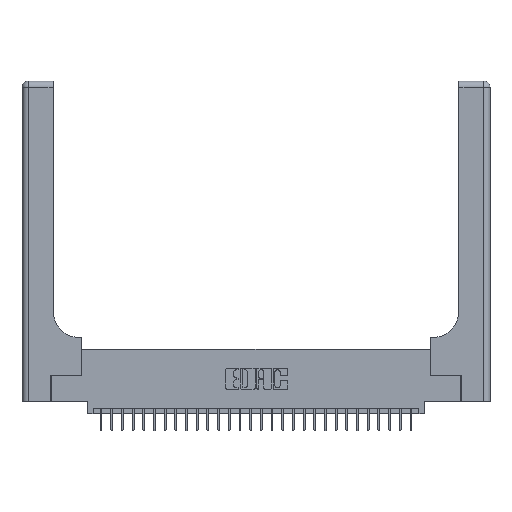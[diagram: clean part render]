
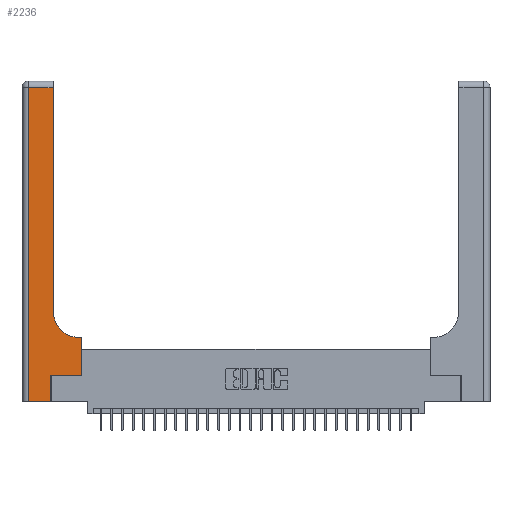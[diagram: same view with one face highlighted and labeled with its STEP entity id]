
A CAD part, top view. The second image highlights one B-rep face of the part: STEP entity #2236.
In plain terms, the highlighted planar face has unit normal (0, 0, 1).
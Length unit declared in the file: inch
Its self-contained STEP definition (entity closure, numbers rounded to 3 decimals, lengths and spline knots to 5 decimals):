
#291 = CARTESIAN_POINT ( 'NONE',  ( 0.06, 2.94, 0.37 ) ) ;
#898 = AXIS2_PLACEMENT_3D ( 'NONE', #12457, #946, #17420 ) ;
#946 = DIRECTION ( 'NONE',  ( 0., 0., -1. ) ) ;
#1152 = CARTESIAN_POINT ( 'NONE',  ( 0.2915, 3., 0.37 ) ) ;
#1405 = CARTESIAN_POINT ( 'NONE',  ( 0.5415, 0.85, 0.37 ) ) ;
#1659 = VECTOR ( 'NONE', #20168, 39.37008 ) ;
#1899 = VERTEX_POINT ( 'NONE', #24719 ) ;
#2165 = LINE ( 'NONE', #14257, #13941 ) ;
#2236 = ADVANCED_FACE ( 'NONE', ( #24741 ), #10393, .F. ) ;
#2517 = LINE ( 'NONE', #11486, #26872 ) ;
#3810 = LINE ( 'NONE', #1152, #28166 ) ;
#3824 = ORIENTED_EDGE ( 'NONE', *, *, #6920, .T. ) ;
#4159 = CARTESIAN_POINT ( 'NONE',  ( 0.269, 0., 0.37 ) ) ;
#4293 = VERTEX_POINT ( 'NONE', #10146 ) ;
#5376 = VERTEX_POINT ( 'NONE', #9492 ) ;
#5674 = EDGE_CURVE ( 'NONE', #18499, #5376, #29000, .T. ) ;
#6738 = EDGE_CURVE ( 'NONE', #12091, #18499, #14197, .T. ) ;
#6920 = EDGE_CURVE ( 'NONE', #1899, #4293, #24886, .T. ) ;
#7078 = DIRECTION ( 'NONE',  ( -1., 0., 0. ) ) ;
#7262 = ORIENTED_EDGE ( 'NONE', *, *, #26365, .T. ) ;
#7520 = EDGE_CURVE ( 'NONE', #28595, #15512, #10056, .T. ) ;
#7571 = CIRCLE ( 'NONE', #26254, 0.25 ) ;
#7953 = CARTESIAN_POINT ( 'NONE',  ( 0.2915, 2.94, 0.37 ) ) ;
#8216 = EDGE_LOOP ( 'NONE', ( #27135, #19461, #10935, #9343, #7262, #21477, #20419, #3824, #23990 ) ) ;
#8591 = DIRECTION ( 'NONE',  ( 1., 0., 0. ) ) ;
#9134 = CARTESIAN_POINT ( 'NONE',  ( 0.269, 0.25, 0.37 ) ) ;
#9343 = ORIENTED_EDGE ( 'NONE', *, *, #10621, .T. ) ;
#9492 = CARTESIAN_POINT ( 'NONE',  ( 0.06, 0., 0.37 ) ) ;
#10056 = LINE ( 'NONE', #9134, #20399 ) ;
#10146 = CARTESIAN_POINT ( 'NONE',  ( 0.5415, 0.6, 0.37 ) ) ;
#10393 = PLANE ( 'NONE',  #898 ) ;
#10621 = EDGE_CURVE ( 'NONE', #5376, #24011, #2165, .T. ) ;
#10935 = ORIENTED_EDGE ( 'NONE', *, *, #5674, .T. ) ;
#11486 = CARTESIAN_POINT ( 'NONE',  ( 0.5585, 0.25, 0.37 ) ) ;
#11944 = DIRECTION ( 'NONE',  ( 1., 0., 0. ) ) ;
#12091 = VERTEX_POINT ( 'NONE', #7953 ) ;
#12300 = VECTOR ( 'NONE', #7078, 39.37008 ) ;
#12457 = CARTESIAN_POINT ( 'NONE',  ( 0., 3., 0.37 ) ) ;
#13941 = VECTOR ( 'NONE', #11944, 39.37008 ) ;
#14134 = EDGE_CURVE ( 'NONE', #15769, #12091, #3810, .T. ) ;
#14197 = LINE ( 'NONE', #17809, #1659 ) ;
#14257 = CARTESIAN_POINT ( 'NONE',  ( 0., 0., 0.37 ) ) ;
#14603 = CARTESIAN_POINT ( 'NONE',  ( 0.06, 3., 0.37 ) ) ;
#15121 = CARTESIAN_POINT ( 'NONE',  ( 0.2915, 0.85, 0.37 ) ) ;
#15512 = VERTEX_POINT ( 'NONE', #30326 ) ;
#15769 = VERTEX_POINT ( 'NONE', #15121 ) ;
#16959 = DIRECTION ( 'NONE',  ( 0., -1., 0. ) ) ;
#17420 = DIRECTION ( 'NONE',  ( -1., 0., 0. ) ) ;
#17809 = CARTESIAN_POINT ( 'NONE',  ( 0., 2.94, 0.37 ) ) ;
#18499 = VERTEX_POINT ( 'NONE', #291 ) ;
#19461 = ORIENTED_EDGE ( 'NONE', *, *, #6738, .T. ) ;
#19994 = DIRECTION ( 'NONE',  ( 0., 1., 0. ) ) ;
#20168 = DIRECTION ( 'NONE',  ( -1., 0., 0. ) ) ;
#20399 = VECTOR ( 'NONE', #26375, 39.37008 ) ;
#20416 = EDGE_CURVE ( 'NONE', #4293, #15769, #7571, .T. ) ;
#20419 = ORIENTED_EDGE ( 'NONE', *, *, #29817, .T. ) ;
#21477 = ORIENTED_EDGE ( 'NONE', *, *, #7520, .T. ) ;
#22551 = CARTESIAN_POINT ( 'NONE',  ( 0.269, 0.25, 0.37 ) ) ;
#23773 = CARTESIAN_POINT ( 'NONE',  ( 0.2915, 0.6, 0.37 ) ) ;
#23813 = VECTOR ( 'NONE', #16959, 39.37008 ) ;
#23990 = ORIENTED_EDGE ( 'NONE', *, *, #20416, .T. ) ;
#24011 = VERTEX_POINT ( 'NONE', #28501 ) ;
#24102 = LINE ( 'NONE', #4159, #30395 ) ;
#24719 = CARTESIAN_POINT ( 'NONE',  ( 0.5585, 0.6, 0.37 ) ) ;
#24741 = FACE_OUTER_BOUND ( 'NONE', #8216, .T. ) ;
#24886 = LINE ( 'NONE', #23773, #12300 ) ;
#26254 = AXIS2_PLACEMENT_3D ( 'NONE', #1405, #29949, #8591 ) ;
#26365 = EDGE_CURVE ( 'NONE', #24011, #28595, #24102, .T. ) ;
#26375 = DIRECTION ( 'NONE',  ( 1., 0., 0. ) ) ;
#26872 = VECTOR ( 'NONE', #29990, 39.37008 ) ;
#27135 = ORIENTED_EDGE ( 'NONE', *, *, #14134, .T. ) ;
#28071 = DIRECTION ( 'NONE',  ( 0., 1., 0. ) ) ;
#28166 = VECTOR ( 'NONE', #19994, 39.37008 ) ;
#28501 = CARTESIAN_POINT ( 'NONE',  ( 0.269, 0., 0.37 ) ) ;
#28595 = VERTEX_POINT ( 'NONE', #22551 ) ;
#29000 = LINE ( 'NONE', #14603, #23813 ) ;
#29817 = EDGE_CURVE ( 'NONE', #15512, #1899, #2517, .T. ) ;
#29949 = DIRECTION ( 'NONE',  ( 0., 0., -1. ) ) ;
#29990 = DIRECTION ( 'NONE',  ( 0., 1., 0. ) ) ;
#30326 = CARTESIAN_POINT ( 'NONE',  ( 0.5585, 0.25, 0.37 ) ) ;
#30395 = VECTOR ( 'NONE', #28071, 39.37008 ) ;
